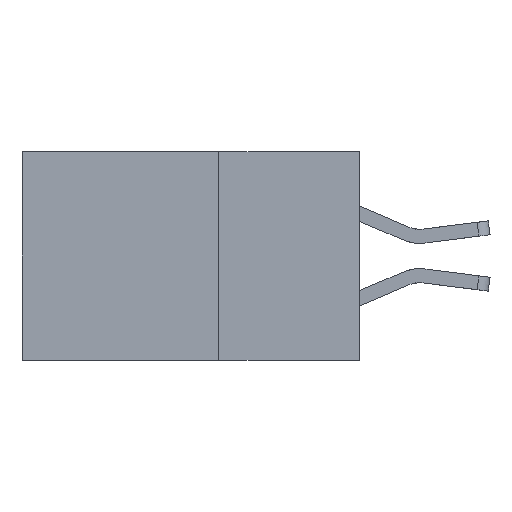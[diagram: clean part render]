
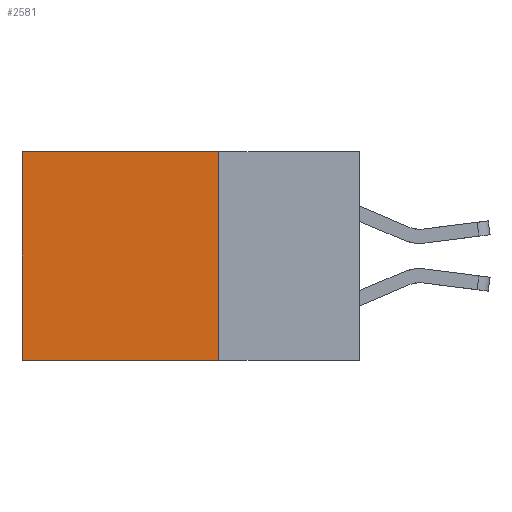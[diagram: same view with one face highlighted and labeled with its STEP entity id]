
A CAD part, left-side view. The second image highlights one B-rep face of the part: STEP entity #2581.
In plain terms, the highlighted planar face has unit normal (-1, 0, 0).
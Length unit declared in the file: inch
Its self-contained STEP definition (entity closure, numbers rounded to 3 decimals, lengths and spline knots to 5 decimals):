
#16 = LINE ( 'NONE', #12770, #7060 ) ;
#668 = EDGE_LOOP ( 'NONE', ( #7790, #9813, #7513, #715 ) ) ;
#715 = ORIENTED_EDGE ( 'NONE', *, *, #3230, .T. ) ;
#730 = EDGE_CURVE ( 'NONE', #7366, #1829, #16, .T. ) ;
#1239 = LINE ( 'NONE', #9277, #3737 ) ;
#1505 = EDGE_CURVE ( 'NONE', #3155, #11555, #1239, .T. ) ;
#1829 = VERTEX_POINT ( 'NONE', #6122 ) ;
#2581 = ADVANCED_FACE ( 'NONE', ( #4499 ), #3019, .F. ) ;
#2732 = DIRECTION ( 'NONE',  ( 0., 0., -1. ) ) ;
#3019 = PLANE ( 'NONE',  #7821 ) ;
#3155 = VERTEX_POINT ( 'NONE', #7127 ) ;
#3191 = LINE ( 'NONE', #12402, #6960 ) ;
#3198 = DIRECTION ( 'NONE',  ( 0., 1., 0. ) ) ;
#3230 = EDGE_CURVE ( 'NONE', #7366, #3155, #11074, .T. ) ;
#3737 = VECTOR ( 'NONE', #12249, 39.37008 ) ;
#4118 = EDGE_CURVE ( 'NONE', #1829, #11555, #3191, .T. ) ;
#4499 = FACE_OUTER_BOUND ( 'NONE', #668, .T. ) ;
#6122 = CARTESIAN_POINT ( 'NONE',  ( 0.2875, 0.25, -0.37 ) ) ;
#6960 = VECTOR ( 'NONE', #3198, 39.37008 ) ;
#6975 = DIRECTION ( 'NONE',  ( 0., 0., -1. ) ) ;
#7060 = VECTOR ( 'NONE', #2732, 39.37008 ) ;
#7127 = CARTESIAN_POINT ( 'NONE',  ( 0.2875, 0.6, 0. ) ) ;
#7366 = VERTEX_POINT ( 'NONE', #12845 ) ;
#7423 = CARTESIAN_POINT ( 'NONE',  ( 0.2875, 0.25, 0. ) ) ;
#7481 = CARTESIAN_POINT ( 'NONE',  ( 0.2875, 0.6, -0.37 ) ) ;
#7513 = ORIENTED_EDGE ( 'NONE', *, *, #730, .F. ) ;
#7790 = ORIENTED_EDGE ( 'NONE', *, *, #1505, .T. ) ;
#7821 = AXIS2_PLACEMENT_3D ( 'NONE', #12136, #9114, #6975 ) ;
#9114 = DIRECTION ( 'NONE',  ( 1., 0., 0. ) ) ;
#9277 = CARTESIAN_POINT ( 'NONE',  ( 0.2875, 0.6, 0. ) ) ;
#9813 = ORIENTED_EDGE ( 'NONE', *, *, #4118, .F. ) ;
#10448 = DIRECTION ( 'NONE',  ( 0., 1., 0. ) ) ;
#10762 = VECTOR ( 'NONE', #10448, 39.37008 ) ;
#11074 = LINE ( 'NONE', #7423, #10762 ) ;
#11555 = VERTEX_POINT ( 'NONE', #7481 ) ;
#12136 = CARTESIAN_POINT ( 'NONE',  ( 0.2875, 0.25, 0. ) ) ;
#12249 = DIRECTION ( 'NONE',  ( 0., 0., -1. ) ) ;
#12402 = CARTESIAN_POINT ( 'NONE',  ( 0.2875, 0.25, -0.37 ) ) ;
#12770 = CARTESIAN_POINT ( 'NONE',  ( 0.2875, 0.25, 0. ) ) ;
#12845 = CARTESIAN_POINT ( 'NONE',  ( 0.2875, 0.25, 0. ) ) ;
